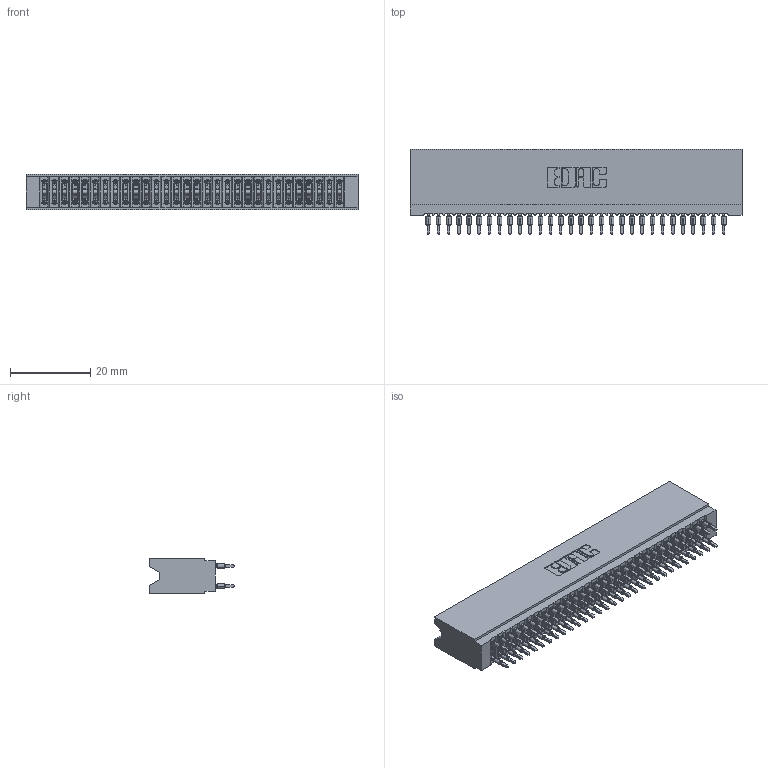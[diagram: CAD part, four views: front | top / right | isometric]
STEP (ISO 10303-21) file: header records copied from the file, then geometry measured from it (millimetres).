
FILE_DESCRIPTION (( 'STEP AP203' ), '1' );
FILE_NAME ('745-060-560-206.STEP', '2026-02-26T19:02:59', ( '' ), ( '' ), 'SwSTEP 2.0', 'SolidWorks 2023', '' );
FILE_SCHEMA (( 'CONFIG_CONTROL_DESIGN' ));
Length unit declared in the file: millimetre
Products named in the file (3): 745-060-560-206; 745 Part_Insulator Option - 06; 745-292-001_560
Assembly tree (61 placements, depth 2):
  745-060-560-206
    745 Part_Insulator Option - 06
    745-292-001_560  x60
Bounding box: 82.8 x 21.22 x 8.89 mm (x, y, z)
Volume: 7729.1 mm3; surface area: 16408.4 mm2
Topology: 61 solids, 61 shells, 6006 faces, 16430 edges, 10432 vertices
Faces by surface type: plane 3116, cylinder 1330, bspline 1200, torus 360
Entity records: 52487 total; most frequent: CARTESIAN_POINT 9612, ORIENTED_EDGE 9024, DIRECTION 7898, EDGE_CURVE 4512, LINE 4142, VECTOR 4142, VERTEX_POINT 2880, AXIS2_PLACEMENT_3D 1878
